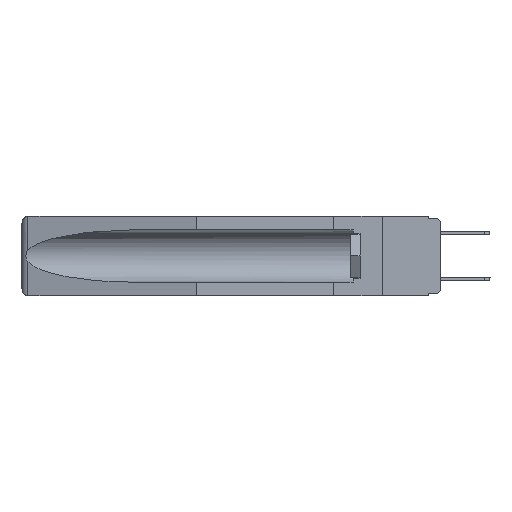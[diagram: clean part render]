
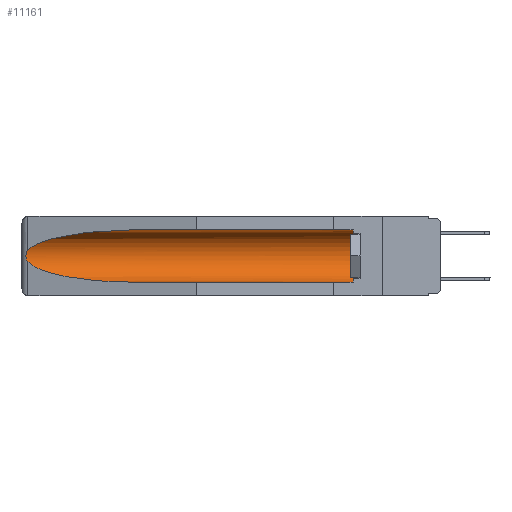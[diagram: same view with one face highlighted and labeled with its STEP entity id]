
A CAD part, left-side view. The second image highlights one B-rep face of the part: STEP entity #11161.
In plain terms, the highlighted cylindrical face has radius 2.857 mm (diameter 5.715 mm), a partial arc.
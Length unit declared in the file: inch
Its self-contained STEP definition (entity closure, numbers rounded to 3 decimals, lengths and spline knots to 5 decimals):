
#396 = CARTESIAN_POINT ( 'NONE',  ( 0.25451, 1.48313, -0.24835 ) ) ;
#543 = VERTEX_POINT ( 'NONE', #857 ) ;
#857 = CARTESIAN_POINT ( 'NONE',  ( 0.155, 1.07973, -0.059 ) ) ;
#994 = CARTESIAN_POINT ( 'NONE',  ( 0.21114, 1.30732, -0.059 ) ) ;
#1308 = DIRECTION ( 'NONE',  ( 0., 1., 0. ) ) ;
#1472 = EDGE_LOOP ( 'NONE', ( #8427, #3567, #2871, #2751, #11024, #10923 ) ) ;
#1684 = DIRECTION ( 'NONE',  ( 0., 1., 0. ) ) ;
#1774 =( BOUNDED_CURVE ( )  B_SPLINE_CURVE ( 3, ( #16609, #994, #8835, #3362 ),
 .UNSPECIFIED., .F., .F. ) 
 B_SPLINE_CURVE_WITH_KNOTS ( ( 4, 4 ),
 ( 4.71239, 6.08839 ),
 .UNSPECIFIED. ) 
 CURVE ( )  GEOMETRIC_REPRESENTATION_ITEM ( )  RATIONAL_B_SPLINE_CURVE ( ( 1., 0.848, 0.848, 1. ) ) 
 REPRESENTATION_ITEM ( '' )  );
#2256 = CARTESIAN_POINT ( 'NONE',  ( 0.26537, 1.52718, -0.19328 ) ) ;
#2420 = DIRECTION ( 'NONE',  ( 0., 0., 1. ) ) ;
#2584 = CARTESIAN_POINT ( 'NONE',  ( 0.26537, 1.52718, -0.14972 ) ) ;
#2751 = ORIENTED_EDGE ( 'NONE', *, *, #12302, .F. ) ;
#2796 = CARTESIAN_POINT ( 'NONE',  ( 0.2675, 1.53308, -0.17534 ) ) ;
#2871 = ORIENTED_EDGE ( 'NONE', *, *, #7174, .T. ) ;
#3006 = VERTEX_POINT ( 'NONE', #15365 ) ;
#3201 = VERTEX_POINT ( 'NONE', #6392 ) ;
#3362 = CARTESIAN_POINT ( 'NONE',  ( 0.26537, 1.52718, -0.14972 ) ) ;
#3567 = ORIENTED_EDGE ( 'NONE', *, *, #9910, .T. ) ;
#3684 = VERTEX_POINT ( 'NONE', #2256 ) ;
#3894 = CARTESIAN_POINT ( 'NONE',  ( 0.2675, 1.53308, -0.16763 ) ) ;
#3952 = B_SPLINE_CURVE_WITH_KNOTS ( 'NONE', 3,
 ( #2584, #9200, #10614, #13176, #3894, #2796, #15707, #9145, #13121, #7928 ),
 .UNSPECIFIED., .F., .F.,
 ( 4, 2, 2, 2, 4 ),
 ( 0., 0.00029, 0.00058, 0.00087, 0.00117 ),
 .UNSPECIFIED. ) ;
#4525 = CARTESIAN_POINT ( 'NONE',  ( 0.155, 0.126, -0.284 ) ) ;
#4811 =( BOUNDED_CURVE ( )  B_SPLINE_CURVE ( 3, ( #8036, #396, #9419, #5436 ),
 .UNSPECIFIED., .F., .F. ) 
 B_SPLINE_CURVE_WITH_KNOTS ( ( 4, 4 ),
 ( 0.1948, 1.5708 ),
 .UNSPECIFIED. ) 
 CURVE ( )  GEOMETRIC_REPRESENTATION_ITEM ( )  RATIONAL_B_SPLINE_CURVE ( ( 1., 0.848, 0.848, 1. ) ) 
 REPRESENTATION_ITEM ( '' )  );
#4883 = EDGE_CURVE ( 'NONE', #3201, #543, #5987, .T. ) ;
#5105 = CARTESIAN_POINT ( 'NONE',  ( 0.155, -0.30754, -0.284 ) ) ;
#5214 = DIRECTION ( 'NONE',  ( 0., 1., 0. ) ) ;
#5385 = DIRECTION ( 'NONE',  ( 0., 0., 1. ) ) ;
#5436 = CARTESIAN_POINT ( 'NONE',  ( 0.155, 1.07973, -0.284 ) ) ;
#5987 = LINE ( 'NONE', #15998, #15933 ) ;
#6392 = CARTESIAN_POINT ( 'NONE',  ( 0.155, 0.126, -0.059 ) ) ;
#6608 = LINE ( 'NONE', #5105, #16547 ) ;
#6650 = DIRECTION ( 'NONE',  ( 0., -1., 0. ) ) ;
#6753 = CARTESIAN_POINT ( 'NONE',  ( 0.155, 0.126, -0.1715 ) ) ;
#7174 = EDGE_CURVE ( 'NONE', #3684, #15740, #4811, .T. ) ;
#7403 = EDGE_CURVE ( 'NONE', #543, #3006, #1774, .T. ) ;
#7705 = FACE_OUTER_BOUND ( 'NONE', #1472, .T. ) ;
#7928 = CARTESIAN_POINT ( 'NONE',  ( 0.26537, 1.52718, -0.19328 ) ) ;
#8036 = CARTESIAN_POINT ( 'NONE',  ( 0.26537, 1.52718, -0.19328 ) ) ;
#8427 = ORIENTED_EDGE ( 'NONE', *, *, #7403, .T. ) ;
#8835 = CARTESIAN_POINT ( 'NONE',  ( 0.25451, 1.48313, -0.09465 ) ) ;
#9145 = CARTESIAN_POINT ( 'NONE',  ( 0.26655, 1.53094, -0.18657 ) ) ;
#9200 = CARTESIAN_POINT ( 'NONE',  ( 0.26597, 1.52961, -0.15275 ) ) ;
#9372 = CIRCLE ( 'NONE', #10070, 0.1125 ) ;
#9419 = CARTESIAN_POINT ( 'NONE',  ( 0.21114, 1.30732, -0.284 ) ) ;
#9910 = EDGE_CURVE ( 'NONE', #3006, #3684, #3952, .T. ) ;
#10070 = AXIS2_PLACEMENT_3D ( 'NONE', #6753, #6650, #5385 ) ;
#10614 = CARTESIAN_POINT ( 'NONE',  ( 0.26654, 1.53092, -0.15636 ) ) ;
#10923 = ORIENTED_EDGE ( 'NONE', *, *, #4883, .T. ) ;
#11024 = ORIENTED_EDGE ( 'NONE', *, *, #14292, .T. ) ;
#11094 = AXIS2_PLACEMENT_3D ( 'NONE', #15840, #1308, #2420 ) ;
#11161 = ADVANCED_FACE ( 'NONE', ( #7705 ), #15033, .F. ) ;
#12302 = EDGE_CURVE ( 'NONE', #14536, #15740, #6608, .T. ) ;
#12840 = CARTESIAN_POINT ( 'NONE',  ( 0.155, 1.07973, -0.284 ) ) ;
#13121 = CARTESIAN_POINT ( 'NONE',  ( 0.26597, 1.5296, -0.19026 ) ) ;
#13176 = CARTESIAN_POINT ( 'NONE',  ( 0.2673, 1.5327, -0.16383 ) ) ;
#14292 = EDGE_CURVE ( 'NONE', #14536, #3201, #9372, .T. ) ;
#14536 = VERTEX_POINT ( 'NONE', #4525 ) ;
#15033 = CYLINDRICAL_SURFACE ( 'NONE', #11094, 0.1125 ) ;
#15365 = CARTESIAN_POINT ( 'NONE',  ( 0.26537, 1.52718, -0.14972 ) ) ;
#15707 = CARTESIAN_POINT ( 'NONE',  ( 0.2673, 1.53269, -0.17917 ) ) ;
#15740 = VERTEX_POINT ( 'NONE', #12840 ) ;
#15840 = CARTESIAN_POINT ( 'NONE',  ( 0.155, -0.30754, -0.1715 ) ) ;
#15933 = VECTOR ( 'NONE', #1684, 39.37008 ) ;
#15998 = CARTESIAN_POINT ( 'NONE',  ( 0.155, -0.30754, -0.059 ) ) ;
#16547 = VECTOR ( 'NONE', #5214, 39.37008 ) ;
#16609 = CARTESIAN_POINT ( 'NONE',  ( 0.155, 1.07973, -0.059 ) ) ;
